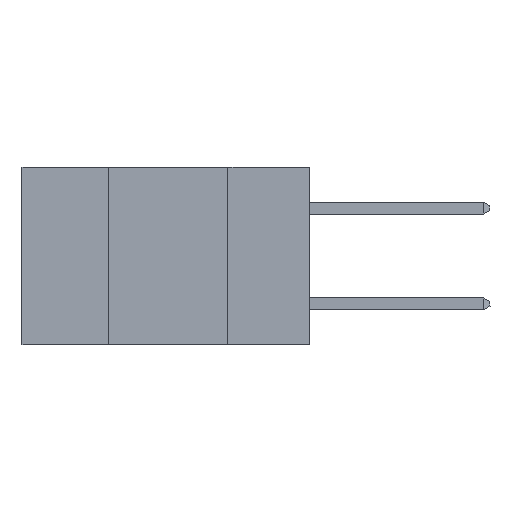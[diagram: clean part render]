
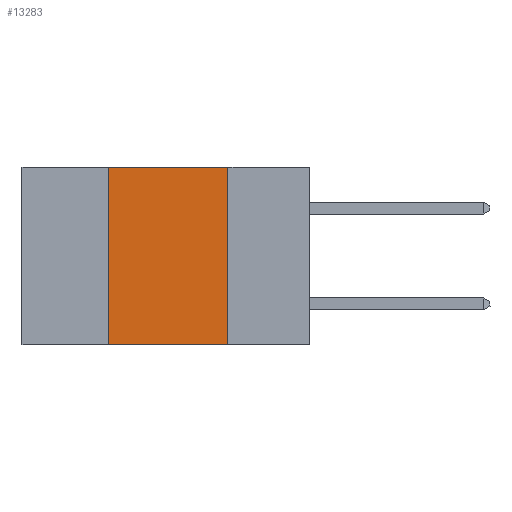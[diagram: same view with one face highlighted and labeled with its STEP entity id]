
A CAD part, left-side view. The second image highlights one B-rep face of the part: STEP entity #13283.
In plain terms, the highlighted planar face has unit normal (-1, 0, 0).
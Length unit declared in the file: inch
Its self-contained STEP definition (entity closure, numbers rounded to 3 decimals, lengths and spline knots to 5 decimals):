
#859 = CARTESIAN_POINT ( 'NONE',  ( 0., 0.17, 0. ) ) ;
#1388 = ORIENTED_EDGE ( 'NONE', *, *, #19975, .T. ) ;
#2015 = VERTEX_POINT ( 'NONE', #9116 ) ;
#2517 = CARTESIAN_POINT ( 'NONE',  ( 0., 0.6, 0. ) ) ;
#2981 = VERTEX_POINT ( 'NONE', #6650 ) ;
#3888 = VECTOR ( 'NONE', #19339, 39.37008 ) ;
#4294 = ORIENTED_EDGE ( 'NONE', *, *, #7403, .F. ) ;
#5677 = LINE ( 'NONE', #9451, #8286 ) ;
#6328 = DIRECTION ( 'NONE',  ( 0., -1., 0. ) ) ;
#6650 = CARTESIAN_POINT ( 'NONE',  ( 0., 0.42, 0. ) ) ;
#6753 = LINE ( 'NONE', #19884, #21262 ) ;
#7403 = EDGE_CURVE ( 'NONE', #2015, #2981, #22213, .T. ) ;
#7414 = PLANE ( 'NONE',  #16602 ) ;
#7464 = VERTEX_POINT ( 'NONE', #859 ) ;
#8286 = VECTOR ( 'NONE', #13176, 39.37008 ) ;
#9039 = DIRECTION ( 'NONE',  ( 1., 0., 0. ) ) ;
#9116 = CARTESIAN_POINT ( 'NONE',  ( 0., 0.42, -0.37 ) ) ;
#9276 = ORIENTED_EDGE ( 'NONE', *, *, #11007, .F. ) ;
#9451 = CARTESIAN_POINT ( 'NONE',  ( 0., 0.6, -0.37 ) ) ;
#11007 = EDGE_CURVE ( 'NONE', #7464, #22915, #6753, .T. ) ;
#12275 = VECTOR ( 'NONE', #6328, 39.37008 ) ;
#13176 = DIRECTION ( 'NONE',  ( 0., -1., 0. ) ) ;
#13283 = ADVANCED_FACE ( 'NONE', ( #16269 ), #7414, .F. ) ;
#13990 = CARTESIAN_POINT ( 'NONE',  ( 0., 0.42, 0. ) ) ;
#14368 = CARTESIAN_POINT ( 'NONE',  ( 0., 0.17, -0.37 ) ) ;
#14377 = DIRECTION ( 'NONE',  ( 0., 0., -1. ) ) ;
#14650 = DIRECTION ( 'NONE',  ( 0., 0., -1. ) ) ;
#16269 = FACE_OUTER_BOUND ( 'NONE', #17156, .T. ) ;
#16602 = AXIS2_PLACEMENT_3D ( 'NONE', #20172, #9039, #14650 ) ;
#17156 = EDGE_LOOP ( 'NONE', ( #9276, #22456, #4294, #1388 ) ) ;
#19339 = DIRECTION ( 'NONE',  ( 0., 0., 1. ) ) ;
#19884 = CARTESIAN_POINT ( 'NONE',  ( 0., 0.17, 0. ) ) ;
#19975 = EDGE_CURVE ( 'NONE', #2015, #22915, #5677, .T. ) ;
#20172 = CARTESIAN_POINT ( 'NONE',  ( 0., 0.6, 0. ) ) ;
#21262 = VECTOR ( 'NONE', #14377, 39.37008 ) ;
#22213 = LINE ( 'NONE', #13990, #3888 ) ;
#22456 = ORIENTED_EDGE ( 'NONE', *, *, #22706, .F. ) ;
#22706 = EDGE_CURVE ( 'NONE', #2981, #7464, #23661, .T. ) ;
#22915 = VERTEX_POINT ( 'NONE', #14368 ) ;
#23661 = LINE ( 'NONE', #2517, #12275 ) ;
